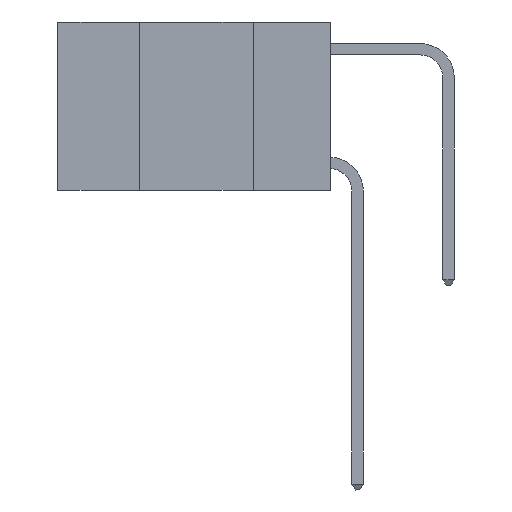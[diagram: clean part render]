
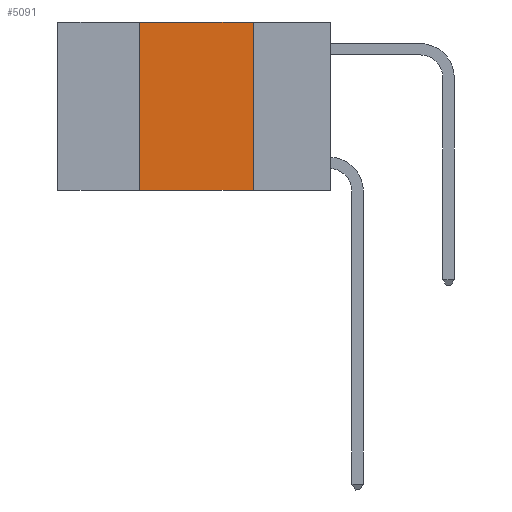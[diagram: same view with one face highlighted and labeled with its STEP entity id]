
A CAD part, left-side view. The second image highlights one B-rep face of the part: STEP entity #5091.
In plain terms, the highlighted planar face has unit normal (-1, 0, 0).
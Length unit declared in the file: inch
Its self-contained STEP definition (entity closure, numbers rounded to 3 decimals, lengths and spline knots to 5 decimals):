
#371 = DIRECTION ( 'NONE',  ( 0., -1., 0. ) ) ;
#504 = DIRECTION ( 'NONE',  ( 0., 0., -1. ) ) ;
#831 = VECTOR ( 'NONE', #10016, 39.37008 ) ;
#993 = VERTEX_POINT ( 'NONE', #7841 ) ;
#1191 = DIRECTION ( 'NONE',  ( 0., 0., -1. ) ) ;
#1234 = VERTEX_POINT ( 'NONE', #7442 ) ;
#1908 = CARTESIAN_POINT ( 'NONE',  ( 0., 0.42, -0.37 ) ) ;
#1915 = CARTESIAN_POINT ( 'NONE',  ( 0., 0.17, -0.37 ) ) ;
#2205 = PLANE ( 'NONE',  #4886 ) ;
#2256 = ORIENTED_EDGE ( 'NONE', *, *, #10336, .F. ) ;
#2304 = EDGE_CURVE ( 'NONE', #10760, #9891, #7366, .T. ) ;
#2421 = VECTOR ( 'NONE', #5795, 39.37008 ) ;
#2724 = EDGE_LOOP ( 'NONE', ( #8391, #7059, #2256, #9826 ) ) ;
#3192 = CARTESIAN_POINT ( 'NONE',  ( 0., 0.42, 0. ) ) ;
#3872 = CARTESIAN_POINT ( 'NONE',  ( 0., 0.6, 0. ) ) ;
#4886 = AXIS2_PLACEMENT_3D ( 'NONE', #3872, #5629, #504 ) ;
#5091 = ADVANCED_FACE ( 'NONE', ( #7176 ), #2205, .F. ) ;
#5629 = DIRECTION ( 'NONE',  ( 1., 0., 0. ) ) ;
#5795 = DIRECTION ( 'NONE',  ( 0., 0., 1. ) ) ;
#6970 = VECTOR ( 'NONE', #1191, 39.37008 ) ;
#7059 = ORIENTED_EDGE ( 'NONE', *, *, #9494, .F. ) ;
#7176 = FACE_OUTER_BOUND ( 'NONE', #2724, .T. ) ;
#7224 = LINE ( 'NONE', #9666, #6970 ) ;
#7366 = LINE ( 'NONE', #8033, #9612 ) ;
#7442 = CARTESIAN_POINT ( 'NONE',  ( 0., 0.42, 0. ) ) ;
#7477 = CARTESIAN_POINT ( 'NONE',  ( 0., 0.6, 0. ) ) ;
#7841 = CARTESIAN_POINT ( 'NONE',  ( 0., 0.17, 0. ) ) ;
#7922 = LINE ( 'NONE', #7477, #831 ) ;
#8033 = CARTESIAN_POINT ( 'NONE',  ( 0., 0.6, -0.37 ) ) ;
#8391 = ORIENTED_EDGE ( 'NONE', *, *, #10862, .F. ) ;
#9226 = LINE ( 'NONE', #3192, #2421 ) ;
#9494 = EDGE_CURVE ( 'NONE', #1234, #993, #7922, .T. ) ;
#9612 = VECTOR ( 'NONE', #371, 39.37008 ) ;
#9666 = CARTESIAN_POINT ( 'NONE',  ( 0., 0.17, 0. ) ) ;
#9826 = ORIENTED_EDGE ( 'NONE', *, *, #2304, .T. ) ;
#9891 = VERTEX_POINT ( 'NONE', #1915 ) ;
#10016 = DIRECTION ( 'NONE',  ( 0., -1., 0. ) ) ;
#10336 = EDGE_CURVE ( 'NONE', #10760, #1234, #9226, .T. ) ;
#10760 = VERTEX_POINT ( 'NONE', #1908 ) ;
#10862 = EDGE_CURVE ( 'NONE', #993, #9891, #7224, .T. ) ;
